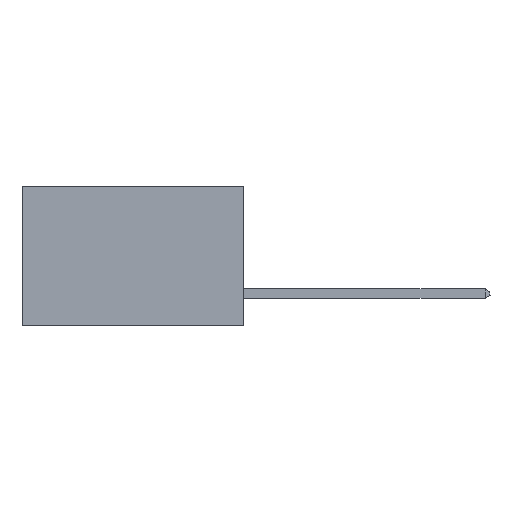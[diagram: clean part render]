
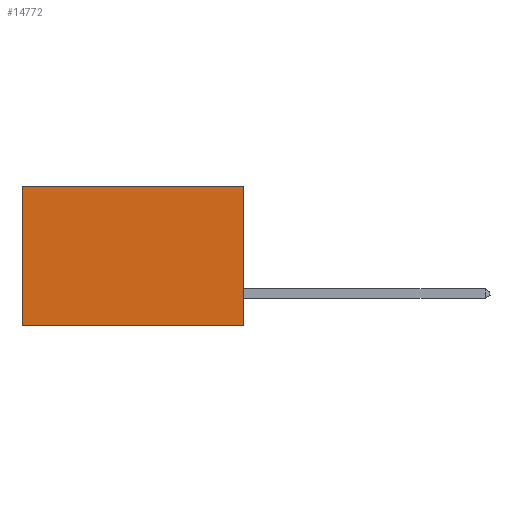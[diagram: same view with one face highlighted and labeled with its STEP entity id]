
A CAD part, left-side view. The second image highlights one B-rep face of the part: STEP entity #14772.
In plain terms, the highlighted planar face has unit normal (-1, 0, 0).
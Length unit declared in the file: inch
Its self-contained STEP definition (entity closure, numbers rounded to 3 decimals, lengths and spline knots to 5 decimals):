
#544 = CARTESIAN_POINT ( 'NONE',  ( 0.277, 0.59, -0.37 ) ) ;
#758 = VECTOR ( 'NONE', #13884, 39.37008 ) ;
#766 = LINE ( 'NONE', #17994, #4582 ) ;
#1578 = VERTEX_POINT ( 'NONE', #544 ) ;
#1993 = CARTESIAN_POINT ( 'NONE',  ( 0.277, 0., -0.37 ) ) ;
#3028 = CARTESIAN_POINT ( 'NONE',  ( 0.277, 0.59, 0. ) ) ;
#3264 = ORIENTED_EDGE ( 'NONE', *, *, #14192, .T. ) ;
#3278 = DIRECTION ( 'NONE',  ( 0., 0., -1. ) ) ;
#3446 = DIRECTION ( 'NONE',  ( 0., 0., -1. ) ) ;
#3741 = CARTESIAN_POINT ( 'NONE',  ( 0.277, 0., -0.37 ) ) ;
#4363 = FACE_OUTER_BOUND ( 'NONE', #14187, .T. ) ;
#4582 = VECTOR ( 'NONE', #15221, 39.37008 ) ;
#5651 = AXIS2_PLACEMENT_3D ( 'NONE', #17611, #12002, #3278 ) ;
#5989 = VECTOR ( 'NONE', #3446, 39.37008 ) ;
#7197 = ORIENTED_EDGE ( 'NONE', *, *, #14976, .F. ) ;
#7667 = ORIENTED_EDGE ( 'NONE', *, *, #17886, .F. ) ;
#8855 = VERTEX_POINT ( 'NONE', #14159 ) ;
#10547 = PLANE ( 'NONE',  #5651 ) ;
#10553 = VECTOR ( 'NONE', #17626, 39.37008 ) ;
#11424 = LINE ( 'NONE', #3741, #758 ) ;
#11997 = VERTEX_POINT ( 'NONE', #12123 ) ;
#12002 = DIRECTION ( 'NONE',  ( 1., 0., 0. ) ) ;
#12123 = CARTESIAN_POINT ( 'NONE',  ( 0.277, 0., -0.37 ) ) ;
#13398 = CARTESIAN_POINT ( 'NONE',  ( 0.277, 0.59, -0.37 ) ) ;
#13685 = LINE ( 'NONE', #1993, #5989 ) ;
#13884 = DIRECTION ( 'NONE',  ( 0., 1., 0. ) ) ;
#14078 = VERTEX_POINT ( 'NONE', #3028 ) ;
#14159 = CARTESIAN_POINT ( 'NONE',  ( 0.277, 0., 0. ) ) ;
#14187 = EDGE_LOOP ( 'NONE', ( #3264, #7197, #7667, #16141 ) ) ;
#14192 = EDGE_CURVE ( 'NONE', #14078, #1578, #15693, .T. ) ;
#14772 = ADVANCED_FACE ( 'NONE', ( #4363 ), #10547, .F. ) ;
#14976 = EDGE_CURVE ( 'NONE', #11997, #1578, #11424, .T. ) ;
#15221 = DIRECTION ( 'NONE',  ( 0., 1., 0. ) ) ;
#15693 = LINE ( 'NONE', #13398, #10553 ) ;
#16141 = ORIENTED_EDGE ( 'NONE', *, *, #17989, .T. ) ;
#17611 = CARTESIAN_POINT ( 'NONE',  ( 0.277, 0., -0.37 ) ) ;
#17626 = DIRECTION ( 'NONE',  ( 0., 0., -1. ) ) ;
#17886 = EDGE_CURVE ( 'NONE', #8855, #11997, #13685, .T. ) ;
#17989 = EDGE_CURVE ( 'NONE', #8855, #14078, #766, .T. ) ;
#17994 = CARTESIAN_POINT ( 'NONE',  ( 0.277, 0., 0. ) ) ;
